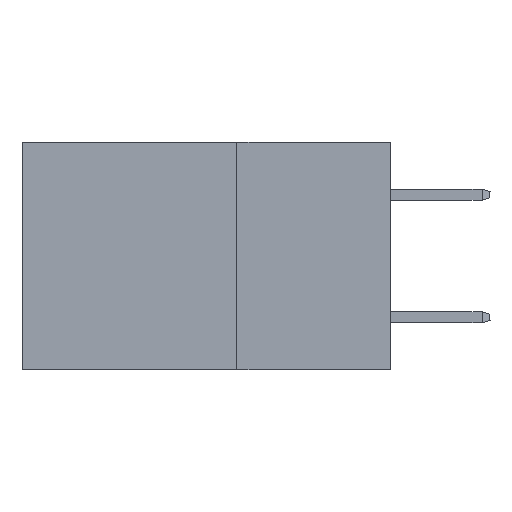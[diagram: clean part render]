
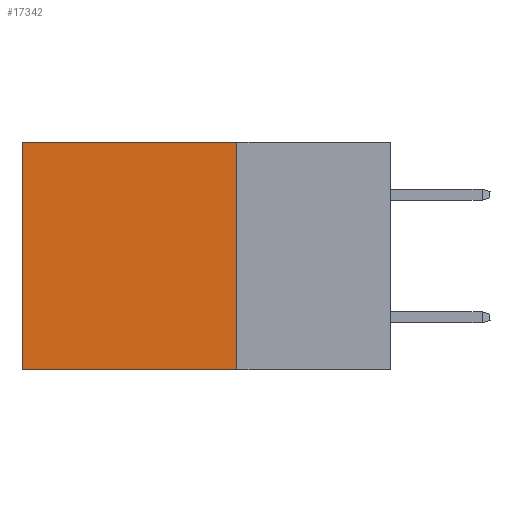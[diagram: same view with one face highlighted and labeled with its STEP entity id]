
A CAD part, left-side view. The second image highlights one B-rep face of the part: STEP entity #17342.
In plain terms, the highlighted planar face has unit normal (-1, 0, 0).
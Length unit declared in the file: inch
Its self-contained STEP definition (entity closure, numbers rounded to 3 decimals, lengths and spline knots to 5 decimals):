
#172 = ORIENTED_EDGE ( 'NONE', *, *, #25000, .F. ) ;
#1464 = DIRECTION ( 'NONE',  ( 0., 0., -1. ) ) ;
#2256 = CARTESIAN_POINT ( 'NONE',  ( 0.2875, 0.25, -0.37 ) ) ;
#2509 = ORIENTED_EDGE ( 'NONE', *, *, #5911, .T. ) ;
#2566 = CARTESIAN_POINT ( 'NONE',  ( 0.2875, 0.25, 0. ) ) ;
#2863 = VERTEX_POINT ( 'NONE', #13275 ) ;
#3321 = VERTEX_POINT ( 'NONE', #14642 ) ;
#4039 = VECTOR ( 'NONE', #15183, 39.37008 ) ;
#5528 = CARTESIAN_POINT ( 'NONE',  ( 0.2875, 0.25, 0. ) ) ;
#5598 = EDGE_LOOP ( 'NONE', ( #27032, #172, #26940, #2509 ) ) ;
#5911 = EDGE_CURVE ( 'NONE', #2863, #3321, #12886, .T. ) ;
#5925 = CARTESIAN_POINT ( 'NONE',  ( 0.2875, 0.6, -0.37 ) ) ;
#6806 = PLANE ( 'NONE',  #14011 ) ;
#9255 = DIRECTION ( 'NONE',  ( 0., 1., 0. ) ) ;
#9545 = FACE_OUTER_BOUND ( 'NONE', #5598, .T. ) ;
#11643 = DIRECTION ( 'NONE',  ( 0., 0., -1. ) ) ;
#12886 = LINE ( 'NONE', #2566, #17564 ) ;
#13258 = DIRECTION ( 'NONE',  ( 0., 0., -1. ) ) ;
#13275 = CARTESIAN_POINT ( 'NONE',  ( 0.2875, 0.25, 0. ) ) ;
#14011 = AXIS2_PLACEMENT_3D ( 'NONE', #23902, #26047, #13258 ) ;
#14642 = CARTESIAN_POINT ( 'NONE',  ( 0.2875, 0.6, 0. ) ) ;
#15183 = DIRECTION ( 'NONE',  ( 0., 1., 0. ) ) ;
#15553 = VECTOR ( 'NONE', #1464, 39.37008 ) ;
#16341 = VERTEX_POINT ( 'NONE', #18658 ) ;
#16952 = EDGE_CURVE ( 'NONE', #3321, #18241, #17577, .T. ) ;
#17342 = ADVANCED_FACE ( 'NONE', ( #9545 ), #6806, .F. ) ;
#17564 = VECTOR ( 'NONE', #9255, 39.37008 ) ;
#17577 = LINE ( 'NONE', #18507, #15553 ) ;
#18241 = VERTEX_POINT ( 'NONE', #5925 ) ;
#18507 = CARTESIAN_POINT ( 'NONE',  ( 0.2875, 0.6, 0. ) ) ;
#18658 = CARTESIAN_POINT ( 'NONE',  ( 0.2875, 0.25, -0.37 ) ) ;
#19673 = VECTOR ( 'NONE', #11643, 39.37008 ) ;
#23795 = LINE ( 'NONE', #2256, #4039 ) ;
#23902 = CARTESIAN_POINT ( 'NONE',  ( 0.2875, 0.25, 0. ) ) ;
#25000 = EDGE_CURVE ( 'NONE', #16341, #18241, #23795, .T. ) ;
#26047 = DIRECTION ( 'NONE',  ( 1., 0., 0. ) ) ;
#26370 = LINE ( 'NONE', #5528, #19673 ) ;
#26787 = EDGE_CURVE ( 'NONE', #2863, #16341, #26370, .T. ) ;
#26940 = ORIENTED_EDGE ( 'NONE', *, *, #26787, .F. ) ;
#27032 = ORIENTED_EDGE ( 'NONE', *, *, #16952, .T. ) ;
